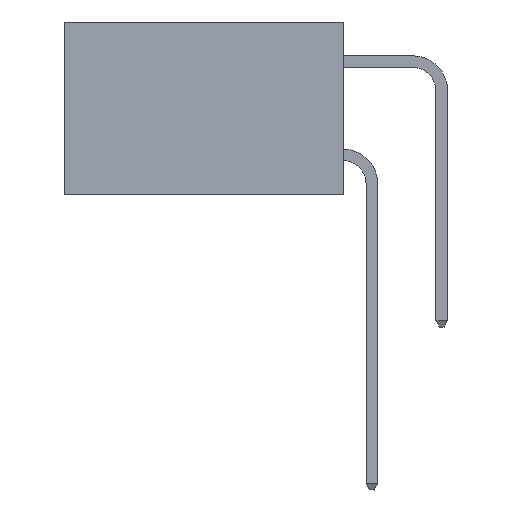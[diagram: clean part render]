
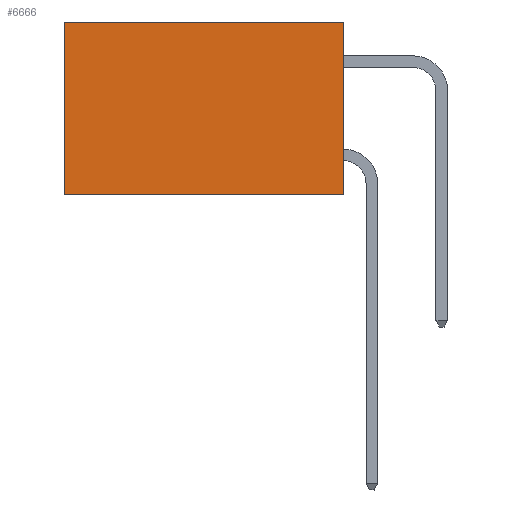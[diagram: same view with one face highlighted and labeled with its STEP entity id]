
A CAD part, left-side view. The second image highlights one B-rep face of the part: STEP entity #6666.
In plain terms, the highlighted planar face has unit normal (-1, 0, 0).
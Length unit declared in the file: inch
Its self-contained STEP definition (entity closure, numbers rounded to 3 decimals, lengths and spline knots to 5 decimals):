
#83 = VECTOR ( 'NONE', #9954, 39.37008 ) ;
#773 = PLANE ( 'NONE',  #14656 ) ;
#1369 = CARTESIAN_POINT ( 'NONE',  ( 0.298, 0.6, 0. ) ) ;
#1386 = VERTEX_POINT ( 'NONE', #15482 ) ;
#1593 = ORIENTED_EDGE ( 'NONE', *, *, #18248, .T. ) ;
#2251 = LINE ( 'NONE', #2336, #14774 ) ;
#2328 = LINE ( 'NONE', #5774, #83 ) ;
#2336 = CARTESIAN_POINT ( 'NONE',  ( 0.298, 0.6, 0. ) ) ;
#3041 = DIRECTION ( 'NONE',  ( 0., 1., 0. ) ) ;
#3517 = EDGE_CURVE ( 'NONE', #5276, #1386, #12380, .T. ) ;
#4333 = EDGE_LOOP ( 'NONE', ( #1593, #5690, #10736, #10314 ) ) ;
#5014 = VECTOR ( 'NONE', #3041, 39.37008 ) ;
#5276 = VERTEX_POINT ( 'NONE', #7456 ) ;
#5690 = ORIENTED_EDGE ( 'NONE', *, *, #3517, .F. ) ;
#5774 = CARTESIAN_POINT ( 'NONE',  ( 0.298, 0., 0. ) ) ;
#6241 = EDGE_CURVE ( 'NONE', #13676, #9469, #2328, .T. ) ;
#6422 = CARTESIAN_POINT ( 'NONE',  ( 0.298, 0., 0. ) ) ;
#6610 = CARTESIAN_POINT ( 'NONE',  ( 0.298, 0., 0. ) ) ;
#6666 = ADVANCED_FACE ( 'NONE', ( #7919 ), #773, .F. ) ;
#7456 = CARTESIAN_POINT ( 'NONE',  ( 0.298, 0., -0.37 ) ) ;
#7919 = FACE_OUTER_BOUND ( 'NONE', #4333, .T. ) ;
#8182 = DIRECTION ( 'NONE',  ( 0., 0., -1. ) ) ;
#9469 = VERTEX_POINT ( 'NONE', #1369 ) ;
#9795 = DIRECTION ( 'NONE',  ( 0., 0., -1. ) ) ;
#9954 = DIRECTION ( 'NONE',  ( 0., 1., 0. ) ) ;
#10139 = VECTOR ( 'NONE', #8182, 39.37008 ) ;
#10314 = ORIENTED_EDGE ( 'NONE', *, *, #6241, .T. ) ;
#10736 = ORIENTED_EDGE ( 'NONE', *, *, #16760, .F. ) ;
#12380 = LINE ( 'NONE', #16882, #5014 ) ;
#13676 = VERTEX_POINT ( 'NONE', #17177 ) ;
#14656 = AXIS2_PLACEMENT_3D ( 'NONE', #6610, #17012, #9795 ) ;
#14774 = VECTOR ( 'NONE', #15362, 39.37008 ) ;
#15362 = DIRECTION ( 'NONE',  ( 0., 0., -1. ) ) ;
#15482 = CARTESIAN_POINT ( 'NONE',  ( 0.298, 0.6, -0.37 ) ) ;
#16760 = EDGE_CURVE ( 'NONE', #13676, #5276, #17540, .T. ) ;
#16882 = CARTESIAN_POINT ( 'NONE',  ( 0.298, 0., -0.37 ) ) ;
#17012 = DIRECTION ( 'NONE',  ( 1., 0., 0. ) ) ;
#17177 = CARTESIAN_POINT ( 'NONE',  ( 0.298, 0., 0. ) ) ;
#17540 = LINE ( 'NONE', #6422, #10139 ) ;
#18248 = EDGE_CURVE ( 'NONE', #9469, #1386, #2251, .T. ) ;
